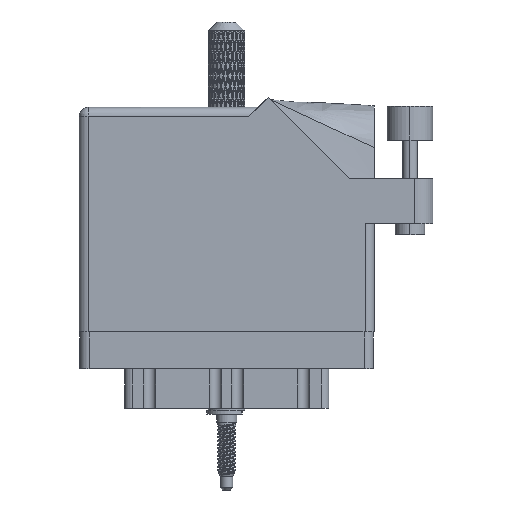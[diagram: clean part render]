
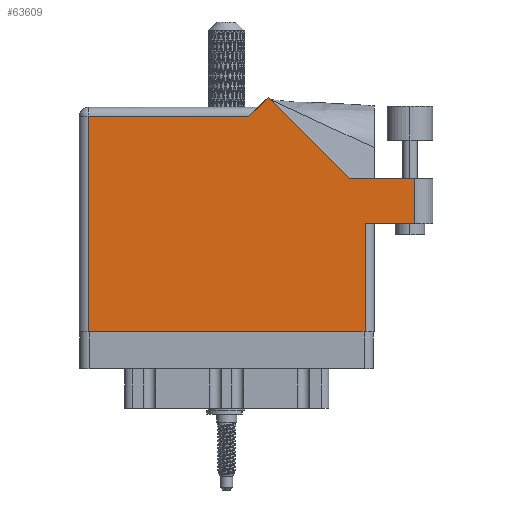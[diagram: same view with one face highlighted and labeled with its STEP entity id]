
A CAD part, front view. The second image highlights one B-rep face of the part: STEP entity #63609.
In plain terms, the highlighted face is planar.
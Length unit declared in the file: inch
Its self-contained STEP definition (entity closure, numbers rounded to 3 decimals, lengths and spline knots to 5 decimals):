
#363 = CARTESIAN_POINT ( 'NONE',  ( 0., 1.468, 0. ) ) ;
#1341 = EDGE_CURVE ( 'NONE', #54797, #7884, #6729, .T. ) ;
#6254 = ORIENTED_EDGE ( 'NONE', *, *, #31333, .T. ) ;
#6729 = LINE ( 'NONE', #103583, #94902 ) ;
#7848 = CARTESIAN_POINT ( 'NONE',  ( 1.948, 0.737, 0. ) ) ;
#7884 = VERTEX_POINT ( 'NONE', #7848 ) ;
#8594 = EDGE_CURVE ( 'NONE', #58493, #72599, #11509, .T. ) ;
#8835 = DIRECTION ( 'NONE',  ( -1., 0., 0. ) ) ;
#11509 = LINE ( 'NONE', #91998, #70928 ) ;
#12048 = DIRECTION ( 'NONE',  ( 0., 1., 0. ) ) ;
#14074 = CARTESIAN_POINT ( 'NONE',  ( 1.84442, 1.044, 0. ) ) ;
#15184 = DIRECTION ( 'NONE',  ( 0., 1., 0. ) ) ;
#15719 = FACE_OUTER_BOUND ( 'NONE', #75046, .T. ) ;
#22408 = CARTESIAN_POINT ( 'NONE',  ( 0.062, 0., 0. ) ) ;
#24156 = CARTESIAN_POINT ( 'NONE',  ( 0., 0., 0. ) ) ;
#28287 = ORIENTED_EDGE ( 'NONE', *, *, #91942, .T. ) ;
#29914 = ORIENTED_EDGE ( 'NONE', *, *, #30162, .T. ) ;
#30162 = EDGE_CURVE ( 'NONE', #92853, #62601, #53405, .T. ) ;
#31333 = EDGE_CURVE ( 'NONE', #72599, #40356, #38620, .T. ) ;
#31703 = CARTESIAN_POINT ( 'NONE',  ( 2.41, 1.044, 0. ) ) ;
#33528 = EDGE_CURVE ( 'NONE', #7884, #58493, #42455, .T. ) ;
#36336 = AXIS2_PLACEMENT_3D ( 'NONE', #103612, #80790, #8835 ) ;
#36933 = ORIENTED_EDGE ( 'NONE', *, *, #67127, .T. ) ;
#37512 = CARTESIAN_POINT ( 'NONE',  ( 1.948, 0., 0. ) ) ;
#38470 = VERTEX_POINT ( 'NONE', #80048 ) ;
#38620 = LINE ( 'NONE', #31703, #43643 ) ;
#40356 = VERTEX_POINT ( 'NONE', #14074 ) ;
#40569 = DIRECTION ( 'NONE',  ( -0.707, -0.707, 0. ) ) ;
#42455 = LINE ( 'NONE', #83196, #47216 ) ;
#42956 = ORIENTED_EDGE ( 'NONE', *, *, #67139, .T. ) ;
#43643 = VECTOR ( 'NONE', #47596, 39.37008 ) ;
#43742 = VECTOR ( 'NONE', #103828, 39.37008 ) ;
#46143 = ORIENTED_EDGE ( 'NONE', *, *, #56953, .T. ) ;
#46976 = VECTOR ( 'NONE', #76235, 39.37008 ) ;
#47216 = VECTOR ( 'NONE', #98598, 39.37008 ) ;
#47596 = DIRECTION ( 'NONE',  ( -1., 0., 0. ) ) ;
#47984 = PLANE ( 'NONE',  #36336 ) ;
#53405 = LINE ( 'NONE', #59296, #46976 ) ;
#54797 = VERTEX_POINT ( 'NONE', #37512 ) ;
#54822 = CARTESIAN_POINT ( 'NONE',  ( 0.062, 1.468, 0. ) ) ;
#55640 = CARTESIAN_POINT ( 'NONE',  ( 1.84442, 1.044, 0. ) ) ;
#56953 = EDGE_CURVE ( 'NONE', #40356, #38470, #96409, .T. ) ;
#58493 = VERTEX_POINT ( 'NONE', #72830 ) ;
#59296 = CARTESIAN_POINT ( 'NONE',  ( 0.062, 0., 0. ) ) ;
#62601 = VERTEX_POINT ( 'NONE', #22408 ) ;
#63379 = ORIENTED_EDGE ( 'NONE', *, *, #1341, .T. ) ;
#63609 = ADVANCED_FACE ( 'NONE', ( #15719 ), #47984, .F. ) ;
#66142 = VERTEX_POINT ( 'NONE', #75048 ) ;
#67127 = EDGE_CURVE ( 'NONE', #66142, #92853, #72853, .T. ) ;
#67139 = EDGE_CURVE ( 'NONE', #62601, #54797, #96697, .T. ) ;
#70928 = VECTOR ( 'NONE', #12048, 39.37008 ) ;
#72599 = VERTEX_POINT ( 'NONE', #100079 ) ;
#72830 = CARTESIAN_POINT ( 'NONE',  ( 2.285, 0.737, 0. ) ) ;
#72853 = LINE ( 'NONE', #363, #74536 ) ;
#74536 = VECTOR ( 'NONE', #98266, 39.37008 ) ;
#75046 = EDGE_LOOP ( 'NONE', ( #82328, #101722, #6254, #46143, #28287, #36933, #29914, #42956, #63379 ) ) ;
#75048 = CARTESIAN_POINT ( 'NONE',  ( 1.155, 1.468, 0. ) ) ;
#76235 = DIRECTION ( 'NONE',  ( 0., -1., 0. ) ) ;
#80048 = CARTESIAN_POINT ( 'NONE',  ( 1.28771, 1.60071, 0. ) ) ;
#80780 = CARTESIAN_POINT ( 'NONE',  ( 1.217, 1.53, 0. ) ) ;
#80790 = DIRECTION ( 'NONE',  ( 0., 0., -1. ) ) ;
#82328 = ORIENTED_EDGE ( 'NONE', *, *, #33528, .T. ) ;
#83196 = CARTESIAN_POINT ( 'NONE',  ( 2.01, 0.737, 0. ) ) ;
#84628 = VECTOR ( 'NONE', #84946, 39.37008 ) ;
#84946 = DIRECTION ( 'NONE',  ( 1., 0., 0. ) ) ;
#88759 = LINE ( 'NONE', #80780, #90618 ) ;
#90618 = VECTOR ( 'NONE', #40569, 39.37008 ) ;
#91942 = EDGE_CURVE ( 'NONE', #38470, #66142, #88759, .T. ) ;
#91998 = CARTESIAN_POINT ( 'NONE',  ( 2.285, 1.044, 0. ) ) ;
#92853 = VERTEX_POINT ( 'NONE', #54822 ) ;
#94902 = VECTOR ( 'NONE', #15184, 39.37008 ) ;
#96409 = LINE ( 'NONE', #55640, #43742 ) ;
#96697 = LINE ( 'NONE', #24156, #84628 ) ;
#98266 = DIRECTION ( 'NONE',  ( -1., 0., 0. ) ) ;
#98598 = DIRECTION ( 'NONE',  ( 1., 0., 0. ) ) ;
#100079 = CARTESIAN_POINT ( 'NONE',  ( 2.285, 1.044, 0. ) ) ;
#101722 = ORIENTED_EDGE ( 'NONE', *, *, #8594, .T. ) ;
#103583 = CARTESIAN_POINT ( 'NONE',  ( 1.948, 0.737, 0. ) ) ;
#103612 = CARTESIAN_POINT ( 'NONE',  ( 0., 1.53, 0. ) ) ;
#103828 = DIRECTION ( 'NONE',  ( -0.707, 0.707, 0. ) ) ;
